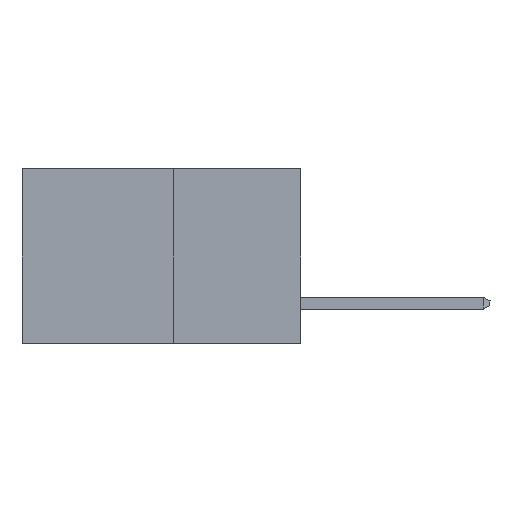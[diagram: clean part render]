
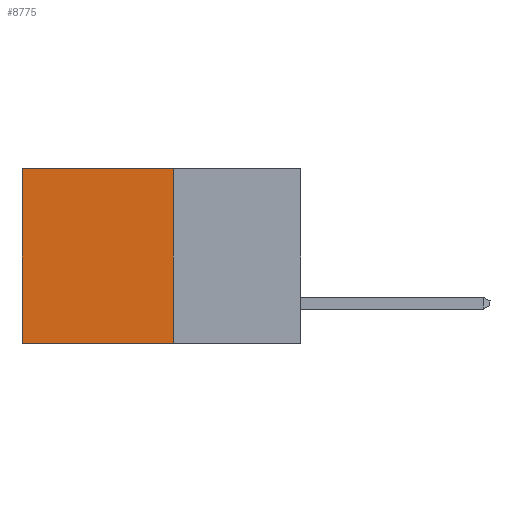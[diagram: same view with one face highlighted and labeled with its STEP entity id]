
A CAD part, left-side view. The second image highlights one B-rep face of the part: STEP entity #8775.
In plain terms, the highlighted planar face has unit normal (-1, 0, 0).
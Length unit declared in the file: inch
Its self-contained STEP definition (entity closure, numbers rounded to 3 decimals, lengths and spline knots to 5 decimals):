
#190 = VERTEX_POINT ( 'NONE', #11555 ) ;
#1518 = DIRECTION ( 'NONE',  ( 0., 0., -1. ) ) ;
#1533 = CARTESIAN_POINT ( 'NONE',  ( 0.277, 0.27, -0.37 ) ) ;
#2663 = LINE ( 'NONE', #11098, #19471 ) ;
#2795 = DIRECTION ( 'NONE',  ( 0., 0., -1. ) ) ;
#3166 = DIRECTION ( 'NONE',  ( 0., 0., -1. ) ) ;
#3518 = ORIENTED_EDGE ( 'NONE', *, *, #13285, .T. ) ;
#4109 = FACE_OUTER_BOUND ( 'NONE', #14653, .T. ) ;
#5359 = VECTOR ( 'NONE', #17716, 39.37008 ) ;
#5662 = VERTEX_POINT ( 'NONE', #7905 ) ;
#5972 = LINE ( 'NONE', #12819, #14103 ) ;
#6067 = CARTESIAN_POINT ( 'NONE',  ( 0.277, 0.59, -0.37 ) ) ;
#6334 = CARTESIAN_POINT ( 'NONE',  ( 0.277, 0.27, -0.37 ) ) ;
#6924 = EDGE_CURVE ( 'NONE', #190, #17881, #6976, .T. ) ;
#6976 = LINE ( 'NONE', #6067, #7487 ) ;
#7487 = VECTOR ( 'NONE', #2795, 39.37008 ) ;
#7905 = CARTESIAN_POINT ( 'NONE',  ( 0.277, 0.27, 0. ) ) ;
#8775 = ADVANCED_FACE ( 'NONE', ( #4109 ), #9624, .F. ) ;
#9384 = EDGE_CURVE ( 'NONE', #18721, #17881, #14003, .T. ) ;
#9624 = PLANE ( 'NONE',  #15335 ) ;
#10076 = ORIENTED_EDGE ( 'NONE', *, *, #13345, .F. ) ;
#11098 = CARTESIAN_POINT ( 'NONE',  ( 0.277, 0.27, 0. ) ) ;
#11555 = CARTESIAN_POINT ( 'NONE',  ( 0.277, 0.59, 0. ) ) ;
#12678 = DIRECTION ( 'NONE',  ( 0., 1., 0. ) ) ;
#12819 = CARTESIAN_POINT ( 'NONE',  ( 0.277, 0.27, -0.37 ) ) ;
#12903 = DIRECTION ( 'NONE',  ( 1., 0., 0. ) ) ;
#13285 = EDGE_CURVE ( 'NONE', #5662, #190, #2663, .T. ) ;
#13345 = EDGE_CURVE ( 'NONE', #5662, #18721, #5972, .T. ) ;
#14003 = LINE ( 'NONE', #6334, #5359 ) ;
#14103 = VECTOR ( 'NONE', #1518, 39.37008 ) ;
#14322 = CARTESIAN_POINT ( 'NONE',  ( 0.277, 0.59, -0.37 ) ) ;
#14653 = EDGE_LOOP ( 'NONE', ( #19999, #15675, #10076, #3518 ) ) ;
#15335 = AXIS2_PLACEMENT_3D ( 'NONE', #1533, #12903, #3166 ) ;
#15675 = ORIENTED_EDGE ( 'NONE', *, *, #9384, .F. ) ;
#17716 = DIRECTION ( 'NONE',  ( 0., 1., 0. ) ) ;
#17881 = VERTEX_POINT ( 'NONE', #14322 ) ;
#18721 = VERTEX_POINT ( 'NONE', #19514 ) ;
#19471 = VECTOR ( 'NONE', #12678, 39.37008 ) ;
#19514 = CARTESIAN_POINT ( 'NONE',  ( 0.277, 0.27, -0.37 ) ) ;
#19999 = ORIENTED_EDGE ( 'NONE', *, *, #6924, .T. ) ;
